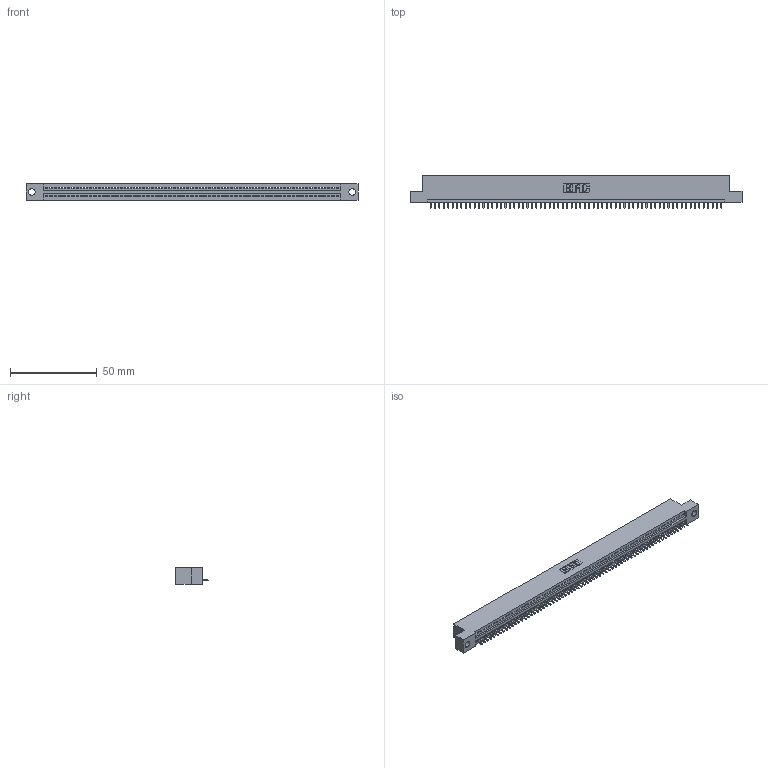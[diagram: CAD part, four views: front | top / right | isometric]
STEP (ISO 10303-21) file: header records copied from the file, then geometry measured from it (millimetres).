
FILE_DESCRIPTION (( 'STEP AP203' ), '1' );
FILE_NAME ('395-067-521-104.STEP', '2021-05-31T22:08:27', ( '' ), ( '' ), 'SwSTEP 2.0', 'SolidWorks 2020', '' );
FILE_SCHEMA (( 'CONFIG_CONTROL_DESIGN' ));
Length unit declared in the file: inch
Products named in the file (3): 345-292-001_345-293-121; 345 Part_Flush Mounting Lugs - 0.156 Dia-TI; 395-067-521-104
Assembly tree (68 placements, depth 2):
  395-067-521-104
    345 Part_Flush Mounting Lugs - 0.156 Dia-TI
    345-292-001_345-293-121  x67
Bounding box: 191.39 x 18.72 x 9.4 mm (x, y, z)
Volume: 18086.5 mm3; surface area: 23472.1 mm2
Topology: 68 solids, 68 shells, 4026 faces, 12169 edges, 8022 vertices
Faces by surface type: plane 2774, cylinder 1252
Entity records: 47497 total; most frequent: CARTESIAN_POINT 8235, ORIENTED_EDGE 8234, DIRECTION 7155, EDGE_CURVE 4117, VECTOR 3717, LINE 3717, VERTEX_POINT 2742, AXIS2_PLACEMENT_3D 1719
